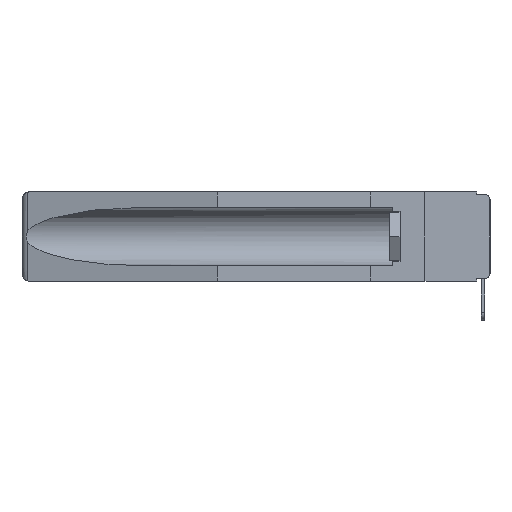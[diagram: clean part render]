
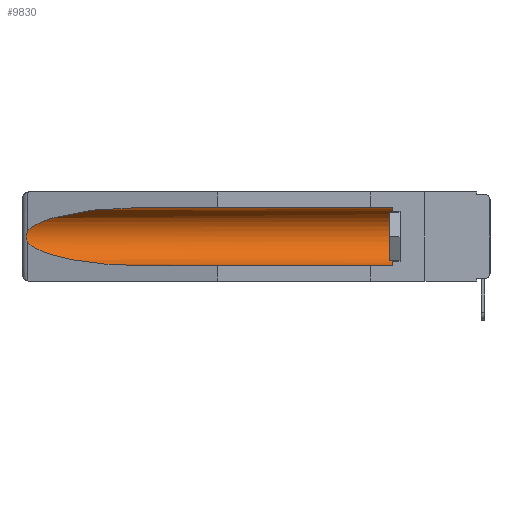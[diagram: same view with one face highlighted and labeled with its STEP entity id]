
A CAD part, left-side view. The second image highlights one B-rep face of the part: STEP entity #9830.
In plain terms, the highlighted cylindrical face has radius 2.857 mm (diameter 5.715 mm), a partial arc.
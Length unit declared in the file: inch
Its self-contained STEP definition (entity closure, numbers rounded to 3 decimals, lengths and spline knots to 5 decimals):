
#164 = CARTESIAN_POINT ( 'NONE',  ( 0.26597, 1.5296, -0.19026 ) ) ;
#1188 = CARTESIAN_POINT ( 'NONE',  ( 0.155, -0.30754, -0.1715 ) ) ;
#1884 = VERTEX_POINT ( 'NONE', #7982 ) ;
#2154 = B_SPLINE_CURVE_WITH_KNOTS ( 'NONE', 3,
 ( #13593, #4216, #14210, #15326, #9985, #4123, #7058, #15497, #164, #16876 ),
 .UNSPECIFIED., .F., .F.,
 ( 4, 2, 2, 2, 4 ),
 ( 0., 0.00029, 0.00058, 0.00087, 0.00117 ),
 .UNSPECIFIED. ) ;
#2367 = CARTESIAN_POINT ( 'NONE',  ( 0.25451, 1.48313, -0.09465 ) ) ;
#2674 = EDGE_CURVE ( 'NONE', #14217, #1884, #10324, .T. ) ;
#3226 = VERTEX_POINT ( 'NONE', #10313 ) ;
#3529 = LINE ( 'NONE', #17664, #13168 ) ;
#3724 = CARTESIAN_POINT ( 'NONE',  ( 0.21114, 1.30732, -0.059 ) ) ;
#3853 = FACE_OUTER_BOUND ( 'NONE', #10136, .T. ) ;
#3969 = ORIENTED_EDGE ( 'NONE', *, *, #17510, .T. ) ;
#4123 = CARTESIAN_POINT ( 'NONE',  ( 0.2675, 1.53308, -0.17534 ) ) ;
#4216 = CARTESIAN_POINT ( 'NONE',  ( 0.26597, 1.52961, -0.15275 ) ) ;
#4501 = CIRCLE ( 'NONE', #6561, 0.1125 ) ;
#5314 = CYLINDRICAL_SURFACE ( 'NONE', #11727, 0.1125 ) ;
#5394 = CARTESIAN_POINT ( 'NONE',  ( 0.155, 0.126, -0.059 ) ) ;
#5410 = EDGE_CURVE ( 'NONE', #12079, #14988, #12381, .T. ) ;
#6296 = DIRECTION ( 'NONE',  ( 0., 1., 0. ) ) ;
#6561 = AXIS2_PLACEMENT_3D ( 'NONE', #11364, #7339, #11460 ) ;
#6599 = DIRECTION ( 'NONE',  ( 0., 1., 0. ) ) ;
#7058 = CARTESIAN_POINT ( 'NONE',  ( 0.2673, 1.53269, -0.17917 ) ) ;
#7124 = CARTESIAN_POINT ( 'NONE',  ( 0.25451, 1.48313, -0.24835 ) ) ;
#7339 = DIRECTION ( 'NONE',  ( 0., -1., 0. ) ) ;
#7403 = CARTESIAN_POINT ( 'NONE',  ( 0.26537, 1.52718, -0.19328 ) ) ;
#7580 = ORIENTED_EDGE ( 'NONE', *, *, #15200, .T. ) ;
#7982 = CARTESIAN_POINT ( 'NONE',  ( 0.155, 1.07973, -0.284 ) ) ;
#8278 = ORIENTED_EDGE ( 'NONE', *, *, #2674, .T. ) ;
#8801 = ORIENTED_EDGE ( 'NONE', *, *, #13098, .T. ) ;
#8805 = EDGE_CURVE ( 'NONE', #3226, #1884, #3529, .T. ) ;
#9830 = ADVANCED_FACE ( 'NONE', ( #3853 ), #5314, .F. ) ;
#9985 = CARTESIAN_POINT ( 'NONE',  ( 0.2675, 1.53308, -0.16763 ) ) ;
#10136 = EDGE_LOOP ( 'NONE', ( #3969, #7580, #8278, #14628, #8801, #14935 ) ) ;
#10288 = CARTESIAN_POINT ( 'NONE',  ( 0.155, 1.07973, -0.059 ) ) ;
#10313 = CARTESIAN_POINT ( 'NONE',  ( 0.155, 0.126, -0.284 ) ) ;
#10324 =( BOUNDED_CURVE ( )  B_SPLINE_CURVE ( 3, ( #7403, #7124, #11427, #11332 ),
 .UNSPECIFIED., .F., .F. ) 
 B_SPLINE_CURVE_WITH_KNOTS ( ( 4, 4 ),
 ( 0.1948, 1.5708 ),
 .UNSPECIFIED. ) 
 CURVE ( )  GEOMETRIC_REPRESENTATION_ITEM ( )  RATIONAL_B_SPLINE_CURVE ( ( 1., 0.848, 0.848, 1. ) ) 
 REPRESENTATION_ITEM ( '' )  );
#10911 = DIRECTION ( 'NONE',  ( 0., 1., 0. ) ) ;
#11031 = VERTEX_POINT ( 'NONE', #13519 ) ;
#11332 = CARTESIAN_POINT ( 'NONE',  ( 0.155, 1.07973, -0.284 ) ) ;
#11364 = CARTESIAN_POINT ( 'NONE',  ( 0.155, 0.126, -0.1715 ) ) ;
#11427 = CARTESIAN_POINT ( 'NONE',  ( 0.21114, 1.30732, -0.284 ) ) ;
#11460 = DIRECTION ( 'NONE',  ( 0., 0., 1. ) ) ;
#11497 =( BOUNDED_CURVE ( )  B_SPLINE_CURVE ( 3, ( #16301, #3724, #2367, #13550 ),
 .UNSPECIFIED., .F., .F. ) 
 B_SPLINE_CURVE_WITH_KNOTS ( ( 4, 4 ),
 ( 4.71239, 6.08839 ),
 .UNSPECIFIED. ) 
 CURVE ( )  GEOMETRIC_REPRESENTATION_ITEM ( )  RATIONAL_B_SPLINE_CURVE ( ( 1., 0.848, 0.848, 1. ) ) 
 REPRESENTATION_ITEM ( '' )  );
#11727 = AXIS2_PLACEMENT_3D ( 'NONE', #1188, #10911, #17623 ) ;
#12063 = CARTESIAN_POINT ( 'NONE',  ( 0.26537, 1.52718, -0.19328 ) ) ;
#12079 = VERTEX_POINT ( 'NONE', #5394 ) ;
#12283 = CARTESIAN_POINT ( 'NONE',  ( 0.155, -0.30754, -0.059 ) ) ;
#12381 = LINE ( 'NONE', #12283, #17820 ) ;
#13098 = EDGE_CURVE ( 'NONE', #3226, #12079, #4501, .T. ) ;
#13168 = VECTOR ( 'NONE', #6296, 39.37008 ) ;
#13519 = CARTESIAN_POINT ( 'NONE',  ( 0.26537, 1.52718, -0.14972 ) ) ;
#13550 = CARTESIAN_POINT ( 'NONE',  ( 0.26537, 1.52718, -0.14972 ) ) ;
#13593 = CARTESIAN_POINT ( 'NONE',  ( 0.26537, 1.52718, -0.14972 ) ) ;
#14210 = CARTESIAN_POINT ( 'NONE',  ( 0.26654, 1.53092, -0.15636 ) ) ;
#14217 = VERTEX_POINT ( 'NONE', #12063 ) ;
#14628 = ORIENTED_EDGE ( 'NONE', *, *, #8805, .F. ) ;
#14935 = ORIENTED_EDGE ( 'NONE', *, *, #5410, .T. ) ;
#14988 = VERTEX_POINT ( 'NONE', #10288 ) ;
#15200 = EDGE_CURVE ( 'NONE', #11031, #14217, #2154, .T. ) ;
#15326 = CARTESIAN_POINT ( 'NONE',  ( 0.2673, 1.5327, -0.16383 ) ) ;
#15497 = CARTESIAN_POINT ( 'NONE',  ( 0.26655, 1.53094, -0.18657 ) ) ;
#16301 = CARTESIAN_POINT ( 'NONE',  ( 0.155, 1.07973, -0.059 ) ) ;
#16876 = CARTESIAN_POINT ( 'NONE',  ( 0.26537, 1.52718, -0.19328 ) ) ;
#17510 = EDGE_CURVE ( 'NONE', #14988, #11031, #11497, .T. ) ;
#17623 = DIRECTION ( 'NONE',  ( 0., 0., 1. ) ) ;
#17664 = CARTESIAN_POINT ( 'NONE',  ( 0.155, -0.30754, -0.284 ) ) ;
#17820 = VECTOR ( 'NONE', #6599, 39.37008 ) ;
